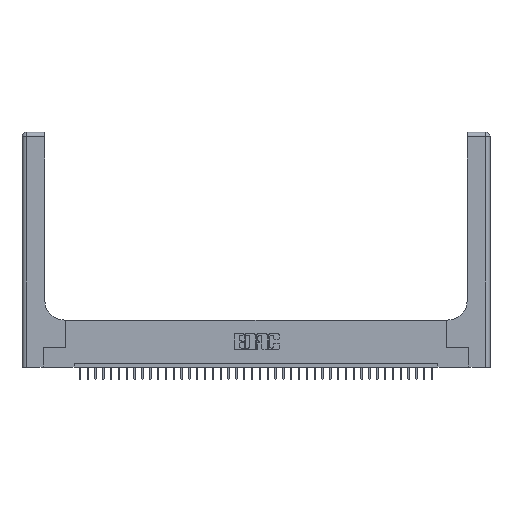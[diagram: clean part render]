
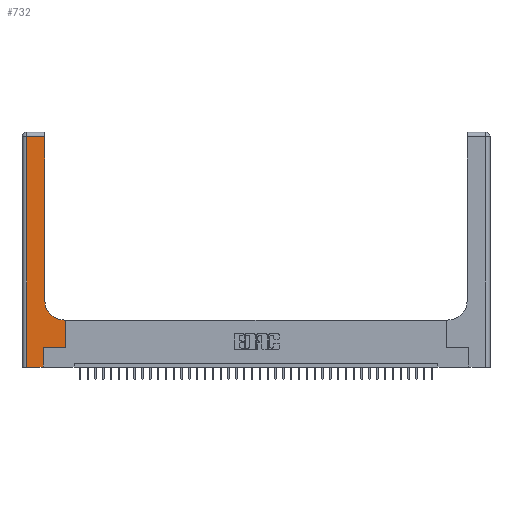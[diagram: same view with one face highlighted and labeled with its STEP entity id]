
A CAD part, top view. The second image highlights one B-rep face of the part: STEP entity #732.
In plain terms, the highlighted planar face has unit normal (0, 0, 1).
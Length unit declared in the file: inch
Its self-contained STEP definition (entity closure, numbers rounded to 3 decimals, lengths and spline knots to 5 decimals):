
#236 = VECTOR ( 'NONE', #25459, 39.37008 ) ;
#732 = ADVANCED_FACE ( 'NONE', ( #12086 ), #35636, .F. ) ;
#1085 = CARTESIAN_POINT ( 'NONE',  ( 0.06, 0., 0.37 ) ) ;
#2537 = CARTESIAN_POINT ( 'NONE',  ( 0.2915, 3., 0.37 ) ) ;
#3284 = ORIENTED_EDGE ( 'NONE', *, *, #3448, .T. ) ;
#3331 = CARTESIAN_POINT ( 'NONE',  ( 0.2915, 0.6, 0.37 ) ) ;
#3448 = EDGE_CURVE ( 'NONE', #31576, #8405, #8061, .T. ) ;
#3502 = EDGE_CURVE ( 'NONE', #21477, #28847, #20930, .T. ) ;
#5364 = CARTESIAN_POINT ( 'NONE',  ( 0.2915, 0.85, 0.37 ) ) ;
#5394 = DIRECTION ( 'NONE',  ( 0., 1., 0. ) ) ;
#5602 = DIRECTION ( 'NONE',  ( -1., 0., 0. ) ) ;
#7705 = LINE ( 'NONE', #2537, #20063 ) ;
#8061 = CIRCLE ( 'NONE', #8547, 0.25 ) ;
#8367 = LINE ( 'NONE', #19333, #236 ) ;
#8405 = VERTEX_POINT ( 'NONE', #5364 ) ;
#8547 = AXIS2_PLACEMENT_3D ( 'NONE', #9198, #35769, #25381 ) ;
#9082 = DIRECTION ( 'NONE',  ( 1., 0., 0. ) ) ;
#9198 = CARTESIAN_POINT ( 'NONE',  ( 0.5415, 0.85, 0.37 ) ) ;
#9772 = CARTESIAN_POINT ( 'NONE',  ( 0.269, 0.25, 0.37 ) ) ;
#9779 = LINE ( 'NONE', #39119, #25550 ) ;
#9974 = CARTESIAN_POINT ( 'NONE',  ( 0.269, 0., 0.37 ) ) ;
#10228 = ORIENTED_EDGE ( 'NONE', *, *, #21557, .T. ) ;
#10704 = VECTOR ( 'NONE', #23767, 39.37008 ) ;
#11244 = ORIENTED_EDGE ( 'NONE', *, *, #27695, .T. ) ;
#12038 = VERTEX_POINT ( 'NONE', #9772 ) ;
#12086 = FACE_OUTER_BOUND ( 'NONE', #23690, .T. ) ;
#13899 = VERTEX_POINT ( 'NONE', #26687 ) ;
#13941 = EDGE_CURVE ( 'NONE', #19797, #12038, #9779, .T. ) ;
#14754 = VECTOR ( 'NONE', #20372, 39.37008 ) ;
#14858 = EDGE_CURVE ( 'NONE', #12038, #21541, #17854, .T. ) ;
#15109 = ORIENTED_EDGE ( 'NONE', *, *, #13941, .T. ) ;
#16176 = LINE ( 'NONE', #36544, #29956 ) ;
#16561 = CARTESIAN_POINT ( 'NONE',  ( 0.06, 3., 0.37 ) ) ;
#17397 = CARTESIAN_POINT ( 'NONE',  ( 0.5585, 0.25, 0.37 ) ) ;
#17854 = LINE ( 'NONE', #24268, #10704 ) ;
#18203 = VECTOR ( 'NONE', #37042, 39.37008 ) ;
#19254 = LINE ( 'NONE', #17397, #27364 ) ;
#19333 = CARTESIAN_POINT ( 'NONE',  ( 0., 2.94, 0.37 ) ) ;
#19468 = CARTESIAN_POINT ( 'NONE',  ( 0.06, 2.94, 0.37 ) ) ;
#19586 = ORIENTED_EDGE ( 'NONE', *, *, #24444, .T. ) ;
#19797 = VERTEX_POINT ( 'NONE', #9974 ) ;
#20063 = VECTOR ( 'NONE', #27140, 39.37008 ) ;
#20372 = DIRECTION ( 'NONE',  ( 0., -1., 0. ) ) ;
#20511 = DIRECTION ( 'NONE',  ( 0., 0., -1. ) ) ;
#20930 = LINE ( 'NONE', #16561, #14754 ) ;
#20959 = AXIS2_PLACEMENT_3D ( 'NONE', #29822, #20511, #5602 ) ;
#21477 = VERTEX_POINT ( 'NONE', #19468 ) ;
#21541 = VERTEX_POINT ( 'NONE', #25744 ) ;
#21557 = EDGE_CURVE ( 'NONE', #13899, #21477, #8367, .T. ) ;
#21878 = ORIENTED_EDGE ( 'NONE', *, *, #14858, .T. ) ;
#23690 = EDGE_LOOP ( 'NONE', ( #27635, #10228, #33139, #19586, #15109, #21878, #26983, #11244, #3284 ) ) ;
#23767 = DIRECTION ( 'NONE',  ( 1., 0., 0. ) ) ;
#24268 = CARTESIAN_POINT ( 'NONE',  ( 0.269, 0.25, 0.37 ) ) ;
#24444 = EDGE_CURVE ( 'NONE', #28847, #19797, #16176, .T. ) ;
#25381 = DIRECTION ( 'NONE',  ( 1., 0., 0. ) ) ;
#25459 = DIRECTION ( 'NONE',  ( -1., 0., 0. ) ) ;
#25550 = VECTOR ( 'NONE', #5394, 39.37008 ) ;
#25744 = CARTESIAN_POINT ( 'NONE',  ( 0.5585, 0.25, 0.37 ) ) ;
#26333 = LINE ( 'NONE', #3331, #18203 ) ;
#26583 = DIRECTION ( 'NONE',  ( 0., 1., 0. ) ) ;
#26610 = VERTEX_POINT ( 'NONE', #31044 ) ;
#26687 = CARTESIAN_POINT ( 'NONE',  ( 0.2915, 2.94, 0.37 ) ) ;
#26983 = ORIENTED_EDGE ( 'NONE', *, *, #33250, .T. ) ;
#27140 = DIRECTION ( 'NONE',  ( 0., 1., 0. ) ) ;
#27364 = VECTOR ( 'NONE', #26583, 39.37008 ) ;
#27635 = ORIENTED_EDGE ( 'NONE', *, *, #28218, .T. ) ;
#27695 = EDGE_CURVE ( 'NONE', #26610, #31576, #26333, .T. ) ;
#27840 = CARTESIAN_POINT ( 'NONE',  ( 0.5415, 0.6, 0.37 ) ) ;
#28218 = EDGE_CURVE ( 'NONE', #8405, #13899, #7705, .T. ) ;
#28847 = VERTEX_POINT ( 'NONE', #1085 ) ;
#29822 = CARTESIAN_POINT ( 'NONE',  ( 0., 3., 0.37 ) ) ;
#29956 = VECTOR ( 'NONE', #9082, 39.37008 ) ;
#31044 = CARTESIAN_POINT ( 'NONE',  ( 0.5585, 0.6, 0.37 ) ) ;
#31576 = VERTEX_POINT ( 'NONE', #27840 ) ;
#33139 = ORIENTED_EDGE ( 'NONE', *, *, #3502, .T. ) ;
#33250 = EDGE_CURVE ( 'NONE', #21541, #26610, #19254, .T. ) ;
#35636 = PLANE ( 'NONE',  #20959 ) ;
#35769 = DIRECTION ( 'NONE',  ( 0., 0., -1. ) ) ;
#36544 = CARTESIAN_POINT ( 'NONE',  ( 0., 0., 0.37 ) ) ;
#37042 = DIRECTION ( 'NONE',  ( -1., 0., 0. ) ) ;
#39119 = CARTESIAN_POINT ( 'NONE',  ( 0.269, 0., 0.37 ) ) ;
